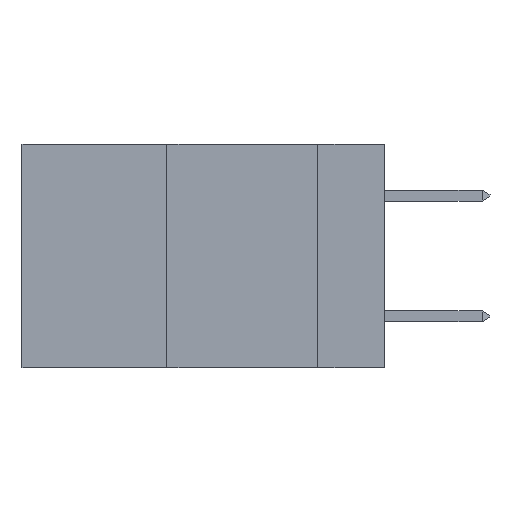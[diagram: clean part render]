
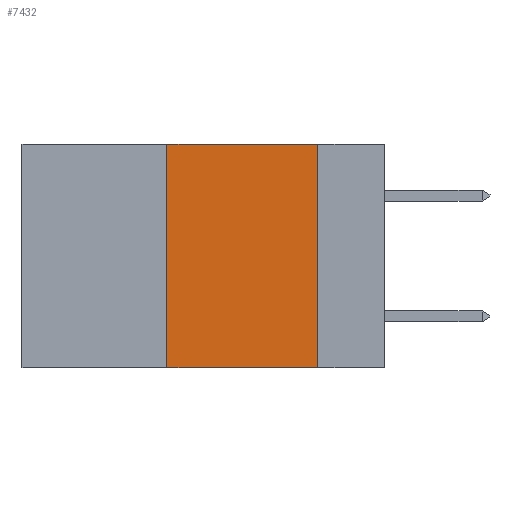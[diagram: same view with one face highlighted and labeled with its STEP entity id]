
A CAD part, left-side view. The second image highlights one B-rep face of the part: STEP entity #7432.
In plain terms, the highlighted planar face has unit normal (-1, 0, 0).
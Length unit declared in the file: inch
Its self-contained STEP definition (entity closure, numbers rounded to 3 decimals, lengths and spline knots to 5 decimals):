
#507 = VECTOR ( 'NONE', #12833, 39.37008 ) ;
#925 = VECTOR ( 'NONE', #4620, 39.37008 ) ;
#1305 = VECTOR ( 'NONE', #12296, 39.37008 ) ;
#1415 = EDGE_LOOP ( 'NONE', ( #4008, #10459, #13446, #1989 ) ) ;
#1663 = LINE ( 'NONE', #5492, #1305 ) ;
#1989 = ORIENTED_EDGE ( 'NONE', *, *, #6501, .T. ) ;
#3005 = DIRECTION ( 'NONE',  ( 1., 0., 0. ) ) ;
#3127 = CARTESIAN_POINT ( 'NONE',  ( 0., 0.36, -0.37 ) ) ;
#3478 = FACE_OUTER_BOUND ( 'NONE', #1415, .T. ) ;
#3647 = LINE ( 'NONE', #8277, #507 ) ;
#4008 = ORIENTED_EDGE ( 'NONE', *, *, #11186, .F. ) ;
#4468 = CARTESIAN_POINT ( 'NONE',  ( 0., 0.11, 0. ) ) ;
#4620 = DIRECTION ( 'NONE',  ( 0., -1., 0. ) ) ;
#5492 = CARTESIAN_POINT ( 'NONE',  ( 0., 0.6, 0. ) ) ;
#5520 = VECTOR ( 'NONE', #13585, 39.37008 ) ;
#5630 = VERTEX_POINT ( 'NONE', #10758 ) ;
#5793 = CARTESIAN_POINT ( 'NONE',  ( 0., 0.11, -0.37 ) ) ;
#5899 = AXIS2_PLACEMENT_3D ( 'NONE', #6423, #3005, #11025 ) ;
#5944 = VERTEX_POINT ( 'NONE', #5793 ) ;
#6423 = CARTESIAN_POINT ( 'NONE',  ( 0., 0.6, 0. ) ) ;
#6501 = EDGE_CURVE ( 'NONE', #13737, #5944, #9421, .T. ) ;
#7432 = ADVANCED_FACE ( 'NONE', ( #3478 ), #9891, .F. ) ;
#8277 = CARTESIAN_POINT ( 'NONE',  ( 0., 0.36, 0. ) ) ;
#9421 = LINE ( 'NONE', #11438, #925 ) ;
#9891 = PLANE ( 'NONE',  #5899 ) ;
#10459 = ORIENTED_EDGE ( 'NONE', *, *, #12457, .F. ) ;
#10758 = CARTESIAN_POINT ( 'NONE',  ( 0., 0.11, 0. ) ) ;
#10889 = CARTESIAN_POINT ( 'NONE',  ( 0., 0.36, 0. ) ) ;
#11025 = DIRECTION ( 'NONE',  ( 0., 0., -1. ) ) ;
#11186 = EDGE_CURVE ( 'NONE', #5630, #5944, #14603, .T. ) ;
#11438 = CARTESIAN_POINT ( 'NONE',  ( 0., 0.6, -0.37 ) ) ;
#12296 = DIRECTION ( 'NONE',  ( 0., -1., 0. ) ) ;
#12457 = EDGE_CURVE ( 'NONE', #14238, #5630, #1663, .T. ) ;
#12833 = DIRECTION ( 'NONE',  ( 0., 0., 1. ) ) ;
#13381 = EDGE_CURVE ( 'NONE', #13737, #14238, #3647, .T. ) ;
#13446 = ORIENTED_EDGE ( 'NONE', *, *, #13381, .F. ) ;
#13585 = DIRECTION ( 'NONE',  ( 0., 0., -1. ) ) ;
#13737 = VERTEX_POINT ( 'NONE', #3127 ) ;
#14238 = VERTEX_POINT ( 'NONE', #10889 ) ;
#14603 = LINE ( 'NONE', #4468, #5520 ) ;
